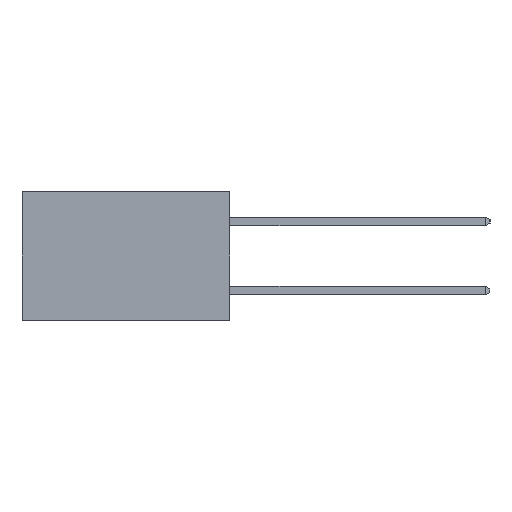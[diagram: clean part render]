
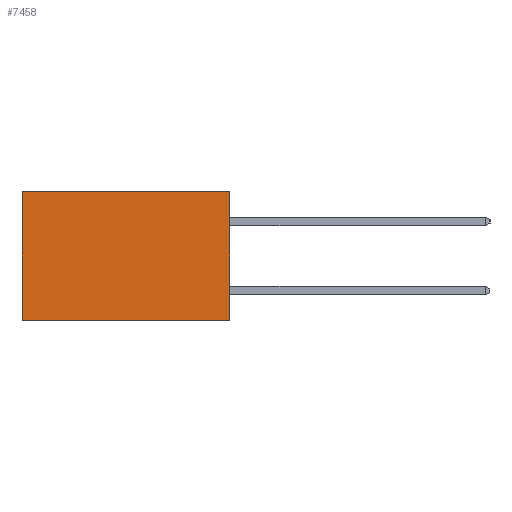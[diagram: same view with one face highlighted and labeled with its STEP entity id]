
A CAD part, left-side view. The second image highlights one B-rep face of the part: STEP entity #7458.
In plain terms, the highlighted planar face has unit normal (-1, 0, 0).
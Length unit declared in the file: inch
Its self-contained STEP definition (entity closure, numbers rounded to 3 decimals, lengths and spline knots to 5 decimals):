
#71 = VERTEX_POINT ( 'NONE', #16472 ) ;
#1161 = VERTEX_POINT ( 'NONE', #22126 ) ;
#3080 = VECTOR ( 'NONE', #17834, 39.37008 ) ;
#3177 = LINE ( 'NONE', #6506, #9461 ) ;
#3736 = LINE ( 'NONE', #15760, #3080 ) ;
#5139 = PLANE ( 'NONE',  #14538 ) ;
#6506 = CARTESIAN_POINT ( 'NONE',  ( 0.298, 0., 0. ) ) ;
#7247 = DIRECTION ( 'NONE',  ( 0., 0., -1. ) ) ;
#7458 = ADVANCED_FACE ( 'NONE', ( #11708 ), #5139, .F. ) ;
#8749 = EDGE_LOOP ( 'NONE', ( #25631, #25545, #23581, #15800 ) ) ;
#9461 = VECTOR ( 'NONE', #21005, 39.37008 ) ;
#9781 = VECTOR ( 'NONE', #17615, 39.37008 ) ;
#11708 = FACE_OUTER_BOUND ( 'NONE', #8749, .T. ) ;
#12206 = CARTESIAN_POINT ( 'NONE',  ( 0.298, 0., 0. ) ) ;
#12239 = LINE ( 'NONE', #12206, #22500 ) ;
#14538 = AXIS2_PLACEMENT_3D ( 'NONE', #15558, #19685, #7247 ) ;
#15365 = EDGE_CURVE ( 'NONE', #71, #1161, #3177, .T. ) ;
#15558 = CARTESIAN_POINT ( 'NONE',  ( 0.298, 0., 0. ) ) ;
#15602 = EDGE_CURVE ( 'NONE', #19273, #16345, #24926, .T. ) ;
#15760 = CARTESIAN_POINT ( 'NONE',  ( 0.298, 0.6, 0. ) ) ;
#15800 = ORIENTED_EDGE ( 'NONE', *, *, #15365, .T. ) ;
#16345 = VERTEX_POINT ( 'NONE', #23611 ) ;
#16472 = CARTESIAN_POINT ( 'NONE',  ( 0.298, 0., 0. ) ) ;
#17615 = DIRECTION ( 'NONE',  ( 0., 1., 0. ) ) ;
#17834 = DIRECTION ( 'NONE',  ( 0., 0., -1. ) ) ;
#19108 = EDGE_CURVE ( 'NONE', #1161, #16345, #3736, .T. ) ;
#19273 = VERTEX_POINT ( 'NONE', #24459 ) ;
#19685 = DIRECTION ( 'NONE',  ( 1., 0., 0. ) ) ;
#20334 = DIRECTION ( 'NONE',  ( 0., 0., -1. ) ) ;
#21005 = DIRECTION ( 'NONE',  ( 0., 1., 0. ) ) ;
#22126 = CARTESIAN_POINT ( 'NONE',  ( 0.298, 0.6, 0. ) ) ;
#22500 = VECTOR ( 'NONE', #20334, 39.37008 ) ;
#23581 = ORIENTED_EDGE ( 'NONE', *, *, #25595, .F. ) ;
#23611 = CARTESIAN_POINT ( 'NONE',  ( 0.298, 0.6, -0.37 ) ) ;
#23702 = CARTESIAN_POINT ( 'NONE',  ( 0.298, 0., -0.37 ) ) ;
#24459 = CARTESIAN_POINT ( 'NONE',  ( 0.298, 0., -0.37 ) ) ;
#24926 = LINE ( 'NONE', #23702, #9781 ) ;
#25545 = ORIENTED_EDGE ( 'NONE', *, *, #15602, .F. ) ;
#25595 = EDGE_CURVE ( 'NONE', #71, #19273, #12239, .T. ) ;
#25631 = ORIENTED_EDGE ( 'NONE', *, *, #19108, .T. ) ;
